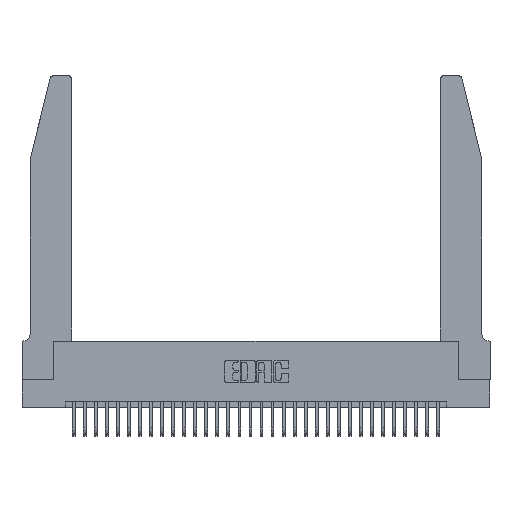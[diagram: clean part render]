
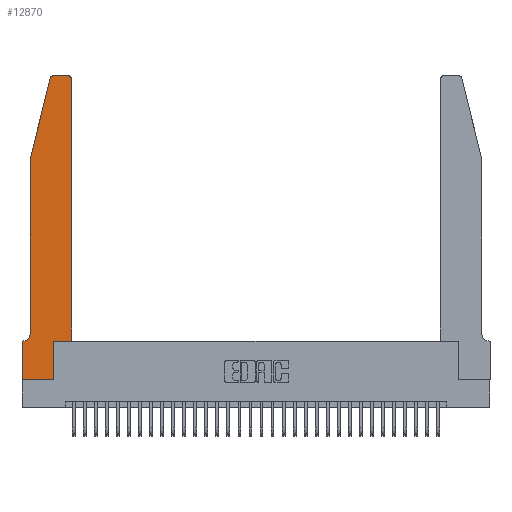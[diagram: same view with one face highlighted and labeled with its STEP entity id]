
A CAD part, top view. The second image highlights one B-rep face of the part: STEP entity #12870.
In plain terms, the highlighted planar face has unit normal (0, 0, 1).
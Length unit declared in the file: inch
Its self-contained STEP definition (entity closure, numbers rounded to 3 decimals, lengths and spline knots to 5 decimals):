
#233 = DIRECTION ( 'NONE',  ( 0., -1., 0. ) ) ;
#252 = VERTEX_POINT ( 'NONE', #13493 ) ;
#447 = EDGE_CURVE ( 'NONE', #29750, #25095, #8347, .T. ) ;
#901 = DIRECTION ( 'NONE',  ( -0.239, -0.971, 0. ) ) ;
#927 = VECTOR ( 'NONE', #10095, 39.37008 ) ;
#1089 = VECTOR ( 'NONE', #26325, 39.37008 ) ;
#1356 = ORIENTED_EDGE ( 'NONE', *, *, #7781, .T. ) ;
#1474 = CARTESIAN_POINT ( 'NONE',  ( 0.2865, 0.35, 0.37 ) ) ;
#1589 = CARTESIAN_POINT ( 'NONE',  ( 0.25487, 2.72718, 0.37 ) ) ;
#2628 = LINE ( 'NONE', #22833, #14842 ) ;
#2804 = CARTESIAN_POINT ( 'NONE',  ( 0.4505, 0.35, 0.37 ) ) ;
#2883 = ORIENTED_EDGE ( 'NONE', *, *, #25599, .T. ) ;
#3448 = DIRECTION ( 'NONE',  ( 0., -1., 0. ) ) ;
#4045 = CARTESIAN_POINT ( 'NONE',  ( 0.0755, 2., 0.37 ) ) ;
#4068 = EDGE_CURVE ( 'NONE', #5189, #29750, #13127, .T. ) ;
#4881 = FACE_OUTER_BOUND ( 'NONE', #22419, .T. ) ;
#5096 = CARTESIAN_POINT ( 'NONE',  ( 0.4205, 2.72, 0.37 ) ) ;
#5189 = VERTEX_POINT ( 'NONE', #30920 ) ;
#5277 = DIRECTION ( 'NONE',  ( 1., 0., 0. ) ) ;
#5524 = VERTEX_POINT ( 'NONE', #5641 ) ;
#5641 = CARTESIAN_POINT ( 'NONE',  ( 0., 0., 0.37 ) ) ;
#5778 = ORIENTED_EDGE ( 'NONE', *, *, #447, .T. ) ;
#6288 = CARTESIAN_POINT ( 'NONE',  ( 0.4205, 2.75, 0.37 ) ) ;
#6730 = ORIENTED_EDGE ( 'NONE', *, *, #17115, .T. ) ;
#7551 = DIRECTION ( 'NONE',  ( 1., 0., 0. ) ) ;
#7648 = CARTESIAN_POINT ( 'NONE',  ( 0.0755, 0.35, 0.37 ) ) ;
#7781 = EDGE_CURVE ( 'NONE', #11064, #16542, #14768, .T. ) ;
#8347 = LINE ( 'NONE', #9337, #1089 ) ;
#8492 = DIRECTION ( 'NONE',  ( 0., 1., 0. ) ) ;
#8732 = VECTOR ( 'NONE', #3448, 39.37008 ) ;
#8748 = DIRECTION ( 'NONE',  ( 0., 0., 1. ) ) ;
#8798 = CARTESIAN_POINT ( 'NONE',  ( 0.284, 2.72, 0.37 ) ) ;
#9337 = CARTESIAN_POINT ( 'NONE',  ( 0.2605, 2.75, 0.37 ) ) ;
#9777 = AXIS2_PLACEMENT_3D ( 'NONE', #23304, #8748, #25737 ) ;
#10051 = ORIENTED_EDGE ( 'NONE', *, *, #19746, .T. ) ;
#10095 = DIRECTION ( 'NONE',  ( -1., 0., 0. ) ) ;
#10758 = EDGE_CURVE ( 'NONE', #252, #28555, #29686, .T. ) ;
#11064 = VERTEX_POINT ( 'NONE', #4045 ) ;
#11071 = VECTOR ( 'NONE', #12502, 39.37008 ) ;
#11210 = DIRECTION ( 'NONE',  ( 1., 0., 0. ) ) ;
#12502 = DIRECTION ( 'NONE',  ( 0., 1., 0. ) ) ;
#12870 = ADVANCED_FACE ( 'NONE', ( #4881 ), #15966, .T. ) ;
#13127 = CIRCLE ( 'NONE', #28348, 0.03 ) ;
#13493 = CARTESIAN_POINT ( 'NONE',  ( 0.2865, 0., 0.37 ) ) ;
#13744 = CARTESIAN_POINT ( 'NONE',  ( 0.0055, 0.42, 0.37 ) ) ;
#14204 = CARTESIAN_POINT ( 'NONE',  ( 0.0055, 0.35, 0.37 ) ) ;
#14273 = VERTEX_POINT ( 'NONE', #14204 ) ;
#14532 = ORIENTED_EDGE ( 'NONE', *, *, #23919, .T. ) ;
#14768 = LINE ( 'NONE', #19749, #20466 ) ;
#14842 = VECTOR ( 'NONE', #901, 39.37008 ) ;
#15966 = PLANE ( 'NONE',  #9777 ) ;
#16175 = DIRECTION ( 'NONE',  ( -1., 0., 0. ) ) ;
#16542 = VERTEX_POINT ( 'NONE', #27707 ) ;
#17115 = EDGE_CURVE ( 'NONE', #5524, #252, #26499, .T. ) ;
#18058 = CARTESIAN_POINT ( 'NONE',  ( 0., 0., 0.37 ) ) ;
#18169 = EDGE_CURVE ( 'NONE', #14273, #19163, #26802, .T. ) ;
#18609 = ORIENTED_EDGE ( 'NONE', *, *, #24004, .T. ) ;
#18854 = AXIS2_PLACEMENT_3D ( 'NONE', #13744, #30678, #16175 ) ;
#18867 = ORIENTED_EDGE ( 'NONE', *, *, #10758, .T. ) ;
#19163 = VERTEX_POINT ( 'NONE', #23666 ) ;
#19746 = EDGE_CURVE ( 'NONE', #16542, #14273, #31202, .T. ) ;
#19749 = CARTESIAN_POINT ( 'NONE',  ( 0.0755, 2., 0.37 ) ) ;
#19765 = LINE ( 'NONE', #2804, #26224 ) ;
#19837 = ORIENTED_EDGE ( 'NONE', *, *, #4068, .T. ) ;
#19931 = CARTESIAN_POINT ( 'NONE',  ( 0.2865, 0.35, 0.37 ) ) ;
#20466 = VECTOR ( 'NONE', #233, 39.37008 ) ;
#20959 = EDGE_CURVE ( 'NONE', #22692, #11064, #2628, .T. ) ;
#22123 = DIRECTION ( 'NONE',  ( 0., 0., 1. ) ) ;
#22419 = EDGE_LOOP ( 'NONE', ( #5778, #18609, #24992, #1356, #10051, #26052, #27813, #6730, #18867, #2883, #14532, #19837 ) ) ;
#22692 = VERTEX_POINT ( 'NONE', #1589 ) ;
#22814 = CARTESIAN_POINT ( 'NONE',  ( 0., 0., 0.37 ) ) ;
#22833 = CARTESIAN_POINT ( 'NONE',  ( 0.0755, 2., 0.37 ) ) ;
#22927 = DIRECTION ( 'NONE',  ( 1., 0., 0. ) ) ;
#23304 = CARTESIAN_POINT ( 'NONE',  ( 0., 0.35, 0.37 ) ) ;
#23308 = VECTOR ( 'NONE', #8492, 39.37008 ) ;
#23666 = CARTESIAN_POINT ( 'NONE',  ( 0., 0.35, 0.37 ) ) ;
#23919 = EDGE_CURVE ( 'NONE', #27366, #5189, #29727, .T. ) ;
#24004 = EDGE_CURVE ( 'NONE', #25095, #22692, #28221, .T. ) ;
#24991 = VECTOR ( 'NONE', #22927, 39.37008 ) ;
#24992 = ORIENTED_EDGE ( 'NONE', *, *, #20959, .T. ) ;
#25095 = VERTEX_POINT ( 'NONE', #28691 ) ;
#25381 = CARTESIAN_POINT ( 'NONE',  ( 0.4505, 0.35, 0.37 ) ) ;
#25599 = EDGE_CURVE ( 'NONE', #28555, #27366, #19765, .T. ) ;
#25737 = DIRECTION ( 'NONE',  ( 1., 0., 0. ) ) ;
#25772 = EDGE_CURVE ( 'NONE', #19163, #5524, #27341, .T. ) ;
#25791 = DIRECTION ( 'NONE',  ( 0., 0., 1. ) ) ;
#26052 = ORIENTED_EDGE ( 'NONE', *, *, #18169, .T. ) ;
#26224 = VECTOR ( 'NONE', #5277, 39.37008 ) ;
#26325 = DIRECTION ( 'NONE',  ( -1., 0., 0. ) ) ;
#26499 = LINE ( 'NONE', #22814, #24991 ) ;
#26802 = LINE ( 'NONE', #7648, #927 ) ;
#27341 = LINE ( 'NONE', #18058, #8732 ) ;
#27366 = VERTEX_POINT ( 'NONE', #29505 ) ;
#27707 = CARTESIAN_POINT ( 'NONE',  ( 0.0755, 0.42, 0.37 ) ) ;
#27813 = ORIENTED_EDGE ( 'NONE', *, *, #25772, .T. ) ;
#28221 = CIRCLE ( 'NONE', #29906, 0.03 ) ;
#28348 = AXIS2_PLACEMENT_3D ( 'NONE', #5096, #22123, #7551 ) ;
#28555 = VERTEX_POINT ( 'NONE', #1474 ) ;
#28691 = CARTESIAN_POINT ( 'NONE',  ( 0.284, 2.75, 0.37 ) ) ;
#29505 = CARTESIAN_POINT ( 'NONE',  ( 0.4505, 0.35, 0.37 ) ) ;
#29686 = LINE ( 'NONE', #19931, #11071 ) ;
#29727 = LINE ( 'NONE', #25381, #23308 ) ;
#29750 = VERTEX_POINT ( 'NONE', #6288 ) ;
#29906 = AXIS2_PLACEMENT_3D ( 'NONE', #8798, #25791, #11210 ) ;
#30678 = DIRECTION ( 'NONE',  ( 0., 0., -1. ) ) ;
#30920 = CARTESIAN_POINT ( 'NONE',  ( 0.4505, 2.72, 0.37 ) ) ;
#31202 = CIRCLE ( 'NONE', #18854, 0.07 ) ;
